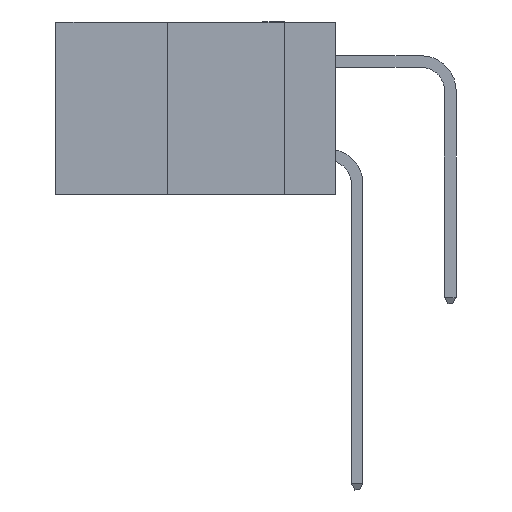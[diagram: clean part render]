
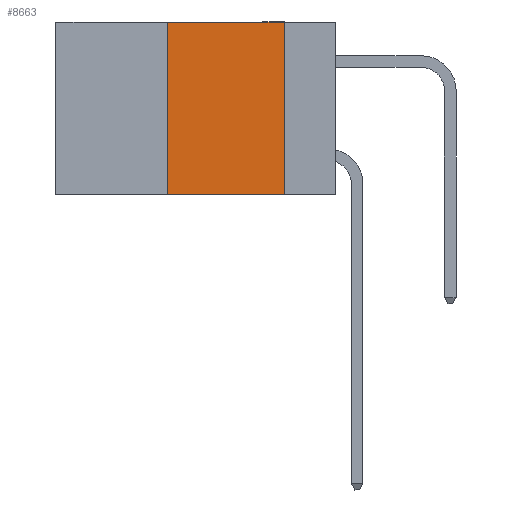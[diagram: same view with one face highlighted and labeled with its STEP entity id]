
A CAD part, left-side view. The second image highlights one B-rep face of the part: STEP entity #8663.
In plain terms, the highlighted planar face has unit normal (-1, 0, 0).
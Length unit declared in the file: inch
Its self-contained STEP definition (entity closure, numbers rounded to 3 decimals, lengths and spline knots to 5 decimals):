
#283 = LINE ( 'NONE', #2477, #14837 ) ;
#350 = CARTESIAN_POINT ( 'NONE',  ( 0., 0.11, -0.37 ) ) ;
#858 = LINE ( 'NONE', #14468, #4860 ) ;
#1971 = CARTESIAN_POINT ( 'NONE',  ( 0., 0.36, 0. ) ) ;
#2323 = AXIS2_PLACEMENT_3D ( 'NONE', #13269, #5394, #6684 ) ;
#2477 = CARTESIAN_POINT ( 'NONE',  ( 0., 0.6, -0.37 ) ) ;
#2608 = DIRECTION ( 'NONE',  ( 0., -1., 0. ) ) ;
#3360 = EDGE_LOOP ( 'NONE', ( #10789, #3529, #15220, #9306 ) ) ;
#3529 = ORIENTED_EDGE ( 'NONE', *, *, #13058, .F. ) ;
#3567 = VERTEX_POINT ( 'NONE', #5364 ) ;
#3615 = LINE ( 'NONE', #13931, #16703 ) ;
#4860 = VECTOR ( 'NONE', #6747, 39.37008 ) ;
#5032 = EDGE_CURVE ( 'NONE', #16336, #15439, #858, .T. ) ;
#5364 = CARTESIAN_POINT ( 'NONE',  ( 0., 0.36, 0. ) ) ;
#5394 = DIRECTION ( 'NONE',  ( 1., 0., 0. ) ) ;
#5934 = FACE_OUTER_BOUND ( 'NONE', #3360, .T. ) ;
#6185 = CARTESIAN_POINT ( 'NONE',  ( 0., 0.36, -0.37 ) ) ;
#6684 = DIRECTION ( 'NONE',  ( 0., 0., -1. ) ) ;
#6747 = DIRECTION ( 'NONE',  ( 0., 0., -1. ) ) ;
#7537 = LINE ( 'NONE', #1971, #7951 ) ;
#7951 = VECTOR ( 'NONE', #15177, 39.37008 ) ;
#8663 = ADVANCED_FACE ( 'NONE', ( #5934 ), #8858, .F. ) ;
#8858 = PLANE ( 'NONE',  #2323 ) ;
#8861 = EDGE_CURVE ( 'NONE', #8980, #3567, #7537, .T. ) ;
#8980 = VERTEX_POINT ( 'NONE', #6185 ) ;
#9306 = ORIENTED_EDGE ( 'NONE', *, *, #13284, .T. ) ;
#9826 = DIRECTION ( 'NONE',  ( 0., -1., 0. ) ) ;
#10789 = ORIENTED_EDGE ( 'NONE', *, *, #5032, .F. ) ;
#13058 = EDGE_CURVE ( 'NONE', #3567, #16336, #3615, .T. ) ;
#13269 = CARTESIAN_POINT ( 'NONE',  ( 0., 0.6, 0. ) ) ;
#13284 = EDGE_CURVE ( 'NONE', #8980, #15439, #283, .T. ) ;
#13479 = CARTESIAN_POINT ( 'NONE',  ( 0., 0.11, 0. ) ) ;
#13931 = CARTESIAN_POINT ( 'NONE',  ( 0., 0.6, 0. ) ) ;
#14468 = CARTESIAN_POINT ( 'NONE',  ( 0., 0.11, 0. ) ) ;
#14837 = VECTOR ( 'NONE', #2608, 39.37008 ) ;
#15177 = DIRECTION ( 'NONE',  ( 0., 0., 1. ) ) ;
#15220 = ORIENTED_EDGE ( 'NONE', *, *, #8861, .F. ) ;
#15439 = VERTEX_POINT ( 'NONE', #350 ) ;
#16336 = VERTEX_POINT ( 'NONE', #13479 ) ;
#16703 = VECTOR ( 'NONE', #9826, 39.37008 ) ;
